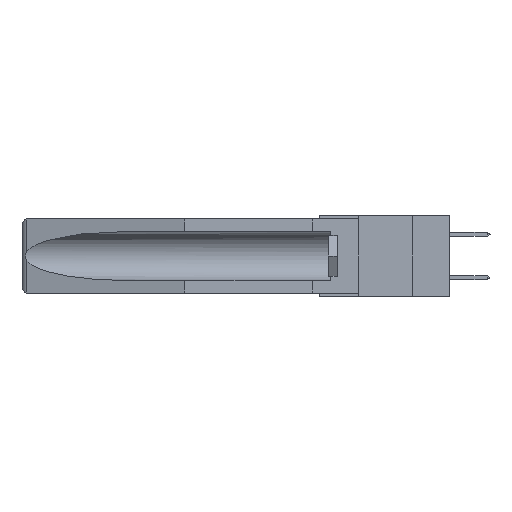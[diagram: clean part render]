
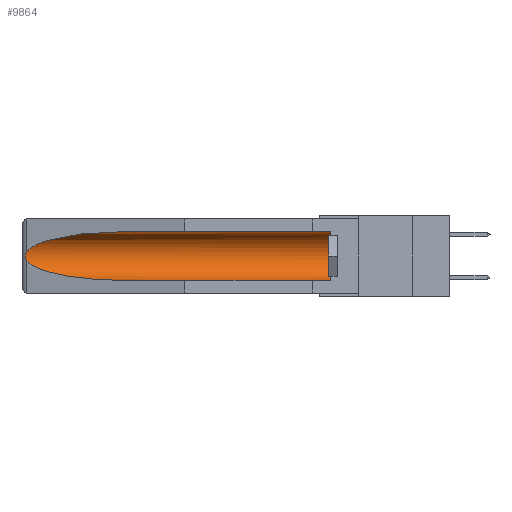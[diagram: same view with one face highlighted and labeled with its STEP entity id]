
A CAD part, left-side view. The second image highlights one B-rep face of the part: STEP entity #9864.
In plain terms, the highlighted cylindrical face has radius 2.857 mm (diameter 5.715 mm), a partial arc.
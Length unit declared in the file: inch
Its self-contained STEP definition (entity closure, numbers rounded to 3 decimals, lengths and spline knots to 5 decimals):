
#1141 = VERTEX_POINT ( 'NONE', #8875 ) ;
#1223 = CARTESIAN_POINT ( 'NONE',  ( 0.26537, 1.52718, -0.14972 ) ) ;
#2174 = VECTOR ( 'NONE', #3576, 39.37008 ) ;
#2437 = DIRECTION ( 'NONE',  ( 0., 1., 0. ) ) ;
#2741 = ORIENTED_EDGE ( 'NONE', *, *, #9305, .T. ) ;
#2766 = AXIS2_PLACEMENT_3D ( 'NONE', #20672, #2437, #18463 ) ;
#3152 =( BOUNDED_CURVE ( )  B_SPLINE_CURVE ( 3, ( #9939, #28391, #33247, #7280 ),
 .UNSPECIFIED., .F., .F. ) 
 B_SPLINE_CURVE_WITH_KNOTS ( ( 4, 4 ),
 ( 0.1948, 1.5708 ),
 .UNSPECIFIED. ) 
 CURVE ( )  GEOMETRIC_REPRESENTATION_ITEM ( )  RATIONAL_B_SPLINE_CURVE ( ( 1., 0.848, 0.848, 1. ) ) 
 REPRESENTATION_ITEM ( '' )  );
#3576 = DIRECTION ( 'NONE',  ( 0., 1., 0. ) ) ;
#3883 = CARTESIAN_POINT ( 'NONE',  ( 0.26597, 1.52961, -0.15275 ) ) ;
#4110 = CARTESIAN_POINT ( 'NONE',  ( 0.2673, 1.5327, -0.16383 ) ) ;
#4556 = CARTESIAN_POINT ( 'NONE',  ( 0.2675, 1.53308, -0.16763 ) ) ;
#5130 = AXIS2_PLACEMENT_3D ( 'NONE', #19666, #30318, #14566 ) ;
#6516 = CARTESIAN_POINT ( 'NONE',  ( 0.26537, 1.52718, -0.14972 ) ) ;
#7280 = CARTESIAN_POINT ( 'NONE',  ( 0.155, 1.07973, -0.284 ) ) ;
#8600 = EDGE_LOOP ( 'NONE', ( #2741, #14886, #12249, #8749, #14782, #16641 ) ) ;
#8749 = ORIENTED_EDGE ( 'NONE', *, *, #31666, .F. ) ;
#8875 = CARTESIAN_POINT ( 'NONE',  ( 0.155, 0.126, -0.284 ) ) ;
#9305 = EDGE_CURVE ( 'NONE', #23543, #13974, #28732, .T. ) ;
#9864 = ADVANCED_FACE ( 'NONE', ( #30646 ), #21246, .F. ) ;
#9939 = CARTESIAN_POINT ( 'NONE',  ( 0.26537, 1.52718, -0.19328 ) ) ;
#9996 = LINE ( 'NONE', #21486, #2174 ) ;
#12249 = ORIENTED_EDGE ( 'NONE', *, *, #27372, .T. ) ;
#12254 = CARTESIAN_POINT ( 'NONE',  ( 0.155, -0.30754, -0.059 ) ) ;
#13636 = VERTEX_POINT ( 'NONE', #23974 ) ;
#13974 = VERTEX_POINT ( 'NONE', #6516 ) ;
#14566 = DIRECTION ( 'NONE',  ( 0., 0., 1. ) ) ;
#14782 = ORIENTED_EDGE ( 'NONE', *, *, #17660, .T. ) ;
#14886 = ORIENTED_EDGE ( 'NONE', *, *, #19004, .T. ) ;
#15409 = CARTESIAN_POINT ( 'NONE',  ( 0.26537, 1.52718, -0.19328 ) ) ;
#16098 = DIRECTION ( 'NONE',  ( 0., 1., 0. ) ) ;
#16641 = ORIENTED_EDGE ( 'NONE', *, *, #25740, .T. ) ;
#17660 = EDGE_CURVE ( 'NONE', #1141, #19182, #18347, .T. ) ;
#18347 = CIRCLE ( 'NONE', #5130, 0.1125 ) ;
#18463 = DIRECTION ( 'NONE',  ( 0., 0., 1. ) ) ;
#19004 = EDGE_CURVE ( 'NONE', #13974, #13636, #26628, .T. ) ;
#19182 = VERTEX_POINT ( 'NONE', #30087 ) ;
#19666 = CARTESIAN_POINT ( 'NONE',  ( 0.155, 0.126, -0.1715 ) ) ;
#20638 = CARTESIAN_POINT ( 'NONE',  ( 0.25451, 1.48313, -0.09465 ) ) ;
#20672 = CARTESIAN_POINT ( 'NONE',  ( 0.155, -0.30754, -0.1715 ) ) ;
#21246 = CYLINDRICAL_SURFACE ( 'NONE', #2766, 0.1125 ) ;
#21486 = CARTESIAN_POINT ( 'NONE',  ( 0.155, -0.30754, -0.284 ) ) ;
#22183 = VERTEX_POINT ( 'NONE', #30835 ) ;
#22569 = CARTESIAN_POINT ( 'NONE',  ( 0.2675, 1.53308, -0.17534 ) ) ;
#23543 = VERTEX_POINT ( 'NONE', #26675 ) ;
#23974 = CARTESIAN_POINT ( 'NONE',  ( 0.26537, 1.52718, -0.19328 ) ) ;
#25671 = CARTESIAN_POINT ( 'NONE',  ( 0.2673, 1.53269, -0.17917 ) ) ;
#25740 = EDGE_CURVE ( 'NONE', #19182, #23543, #32006, .T. ) ;
#25794 = CARTESIAN_POINT ( 'NONE',  ( 0.26537, 1.52718, -0.14972 ) ) ;
#26335 = VECTOR ( 'NONE', #16098, 39.37008 ) ;
#26628 = B_SPLINE_CURVE_WITH_KNOTS ( 'NONE', 3,
 ( #1223, #3883, #30803, #4110, #4556, #22569, #25671, #31124, #33516, #15409 ),
 .UNSPECIFIED., .F., .F.,
 ( 4, 2, 2, 2, 4 ),
 ( 0., 0.00029, 0.00058, 0.00087, 0.00117 ),
 .UNSPECIFIED. ) ;
#26675 = CARTESIAN_POINT ( 'NONE',  ( 0.155, 1.07973, -0.059 ) ) ;
#27372 = EDGE_CURVE ( 'NONE', #13636, #22183, #3152, .T. ) ;
#28094 = CARTESIAN_POINT ( 'NONE',  ( 0.21114, 1.30732, -0.059 ) ) ;
#28391 = CARTESIAN_POINT ( 'NONE',  ( 0.25451, 1.48313, -0.24835 ) ) ;
#28439 = CARTESIAN_POINT ( 'NONE',  ( 0.155, 1.07973, -0.059 ) ) ;
#28732 =( BOUNDED_CURVE ( )  B_SPLINE_CURVE ( 3, ( #28439, #28094, #20638, #25794 ),
 .UNSPECIFIED., .F., .F. ) 
 B_SPLINE_CURVE_WITH_KNOTS ( ( 4, 4 ),
 ( 4.71239, 6.08839 ),
 .UNSPECIFIED. ) 
 CURVE ( )  GEOMETRIC_REPRESENTATION_ITEM ( )  RATIONAL_B_SPLINE_CURVE ( ( 1., 0.848, 0.848, 1. ) ) 
 REPRESENTATION_ITEM ( '' )  );
#30087 = CARTESIAN_POINT ( 'NONE',  ( 0.155, 0.126, -0.059 ) ) ;
#30318 = DIRECTION ( 'NONE',  ( 0., -1., 0. ) ) ;
#30646 = FACE_OUTER_BOUND ( 'NONE', #8600, .T. ) ;
#30803 = CARTESIAN_POINT ( 'NONE',  ( 0.26654, 1.53092, -0.15636 ) ) ;
#30835 = CARTESIAN_POINT ( 'NONE',  ( 0.155, 1.07973, -0.284 ) ) ;
#31124 = CARTESIAN_POINT ( 'NONE',  ( 0.26655, 1.53094, -0.18657 ) ) ;
#31666 = EDGE_CURVE ( 'NONE', #1141, #22183, #9996, .T. ) ;
#32006 = LINE ( 'NONE', #12254, #26335 ) ;
#33247 = CARTESIAN_POINT ( 'NONE',  ( 0.21114, 1.30732, -0.284 ) ) ;
#33516 = CARTESIAN_POINT ( 'NONE',  ( 0.26597, 1.5296, -0.19026 ) ) ;
